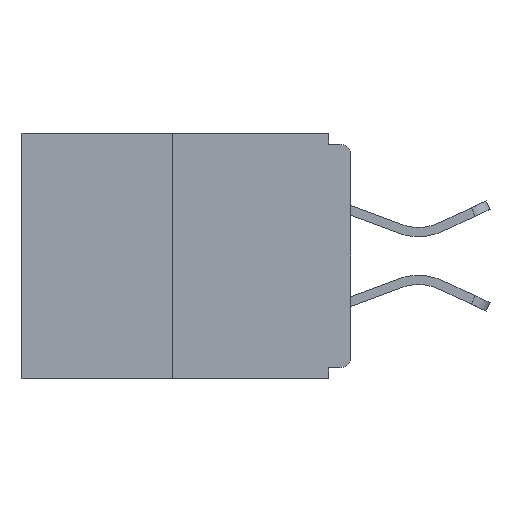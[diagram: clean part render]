
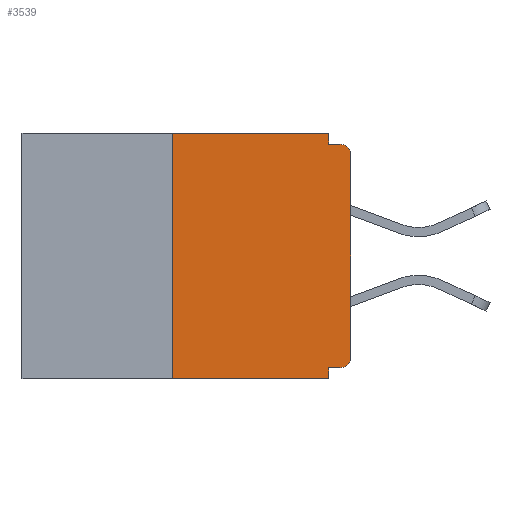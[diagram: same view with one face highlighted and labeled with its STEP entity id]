
A CAD part, left-side view. The second image highlights one B-rep face of the part: STEP entity #3539.
In plain terms, the highlighted planar face has unit normal (-1, 0, 0).
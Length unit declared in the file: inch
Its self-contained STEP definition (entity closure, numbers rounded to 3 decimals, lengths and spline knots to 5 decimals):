
#502 = CARTESIAN_POINT ( 'NONE',  ( 0., 0.46, 0. ) ) ;
#563 = EDGE_CURVE ( 'NONE', #7526, #619, #7329, .T. ) ;
#617 = CARTESIAN_POINT ( 'NONE',  ( 0., 0., 0. ) ) ;
#619 = VERTEX_POINT ( 'NONE', #12377 ) ;
#765 = DIRECTION ( 'NONE',  ( 0., 0., 1. ) ) ;
#1009 = CARTESIAN_POINT ( 'NONE',  ( 0., 0.031, -0.343 ) ) ;
#1024 = EDGE_CURVE ( 'NONE', #7980, #8264, #1423, .T. ) ;
#1290 = ORIENTED_EDGE ( 'NONE', *, *, #9973, .T. ) ;
#1423 = CIRCLE ( 'NONE', #4013, 0.015 ) ;
#1429 = CARTESIAN_POINT ( 'NONE',  ( 0., 0.031, -0.343 ) ) ;
#1476 = ORIENTED_EDGE ( 'NONE', *, *, #5410, .F. ) ;
#1592 = VECTOR ( 'NONE', #1594, 39.37008 ) ;
#1594 = DIRECTION ( 'NONE',  ( 0., 1., 0. ) ) ;
#1941 = DIRECTION ( 'NONE',  ( -1., 0., 0. ) ) ;
#1997 = CARTESIAN_POINT ( 'NONE',  ( 0., 0.46, -0.343 ) ) ;
#2198 = CARTESIAN_POINT ( 'NONE',  ( 0., 0.031, 0. ) ) ;
#2380 = VECTOR ( 'NONE', #7196, 39.37008 ) ;
#2473 = CARTESIAN_POINT ( 'NONE',  ( 0., 0.015, -0.328 ) ) ;
#2651 = VERTEX_POINT ( 'NONE', #6211 ) ;
#2707 = VECTOR ( 'NONE', #7493, 39.37008 ) ;
#2722 = DIRECTION ( 'NONE',  ( 0., -1., 0. ) ) ;
#2783 = LINE ( 'NONE', #9301, #4203 ) ;
#2908 = CARTESIAN_POINT ( 'NONE',  ( 0., 0., -0.03 ) ) ;
#3265 = PLANE ( 'NONE',  #10015 ) ;
#3532 = CARTESIAN_POINT ( 'NONE',  ( 0., 0.015, -0.015 ) ) ;
#3539 = ADVANCED_FACE ( 'NONE', ( #5276 ), #3265, .F. ) ;
#3884 = ORIENTED_EDGE ( 'NONE', *, *, #563, .F. ) ;
#3945 = CARTESIAN_POINT ( 'NONE',  ( 0., 0.015, -0.03 ) ) ;
#3946 = CARTESIAN_POINT ( 'NONE',  ( 0., 0.031, 0. ) ) ;
#4000 = ORIENTED_EDGE ( 'NONE', *, *, #6491, .F. ) ;
#4013 = AXIS2_PLACEMENT_3D ( 'NONE', #5721, #1941, #5534 ) ;
#4203 = VECTOR ( 'NONE', #2722, 39.37008 ) ;
#4237 = CARTESIAN_POINT ( 'NONE',  ( 0., 0.031, -0.015 ) ) ;
#4434 = VERTEX_POINT ( 'NONE', #2198 ) ;
#4523 = EDGE_CURVE ( 'NONE', #619, #4434, #6248, .T. ) ;
#4930 = VECTOR ( 'NONE', #6283, 39.37008 ) ;
#5276 = FACE_OUTER_BOUND ( 'NONE', #11549, .T. ) ;
#5347 = CARTESIAN_POINT ( 'NONE',  ( 0., 0.46, 0. ) ) ;
#5410 = EDGE_CURVE ( 'NONE', #4434, #6881, #11547, .T. ) ;
#5431 = VERTEX_POINT ( 'NONE', #1009 ) ;
#5495 = CARTESIAN_POINT ( 'NONE',  ( 0., 0.25, -0.343 ) ) ;
#5534 = DIRECTION ( 'NONE',  ( 0., 0., -1. ) ) ;
#5581 = EDGE_CURVE ( 'NONE', #8264, #8091, #8442, .T. ) ;
#5721 = CARTESIAN_POINT ( 'NONE',  ( 0., 0.015, -0.313 ) ) ;
#5841 = LINE ( 'NONE', #1997, #8376 ) ;
#6211 = CARTESIAN_POINT ( 'NONE',  ( 0., 0.031, -0.328 ) ) ;
#6248 = LINE ( 'NONE', #502, #2380 ) ;
#6283 = DIRECTION ( 'NONE',  ( 0., 0., -1. ) ) ;
#6317 = EDGE_CURVE ( 'NONE', #7526, #5431, #5841, .T. ) ;
#6377 = CARTESIAN_POINT ( 'NONE',  ( 0., 0.25, 0. ) ) ;
#6491 = EDGE_CURVE ( 'NONE', #2651, #5431, #7106, .T. ) ;
#6863 = ORIENTED_EDGE ( 'NONE', *, *, #1024, .T. ) ;
#6881 = VERTEX_POINT ( 'NONE', #4237 ) ;
#6910 = VERTEX_POINT ( 'NONE', #3532 ) ;
#7106 = LINE ( 'NONE', #1429, #4930 ) ;
#7196 = DIRECTION ( 'NONE',  ( 0., -1., 0. ) ) ;
#7329 = LINE ( 'NONE', #6377, #10081 ) ;
#7493 = DIRECTION ( 'NONE',  ( 0., 0., 1. ) ) ;
#7526 = VERTEX_POINT ( 'NONE', #5495 ) ;
#7821 = DIRECTION ( 'NONE',  ( 0., 0., -1. ) ) ;
#7980 = VERTEX_POINT ( 'NONE', #2473 ) ;
#8091 = VERTEX_POINT ( 'NONE', #2908 ) ;
#8264 = VERTEX_POINT ( 'NONE', #10999 ) ;
#8376 = VECTOR ( 'NONE', #10748, 39.37008 ) ;
#8391 = LINE ( 'NONE', #9409, #1592 ) ;
#8442 = LINE ( 'NONE', #617, #2707 ) ;
#8586 = CIRCLE ( 'NONE', #9596, 0.015 ) ;
#9151 = DIRECTION ( 'NONE',  ( 0., 0., -1. ) ) ;
#9166 = ORIENTED_EDGE ( 'NONE', *, *, #9200, .F. ) ;
#9200 = EDGE_CURVE ( 'NONE', #7980, #2651, #8391, .T. ) ;
#9216 = VECTOR ( 'NONE', #7821, 39.37008 ) ;
#9301 = CARTESIAN_POINT ( 'NONE',  ( 0., 0., -0.015 ) ) ;
#9409 = CARTESIAN_POINT ( 'NONE',  ( 0., 0., -0.328 ) ) ;
#9530 = ORIENTED_EDGE ( 'NONE', *, *, #5581, .T. ) ;
#9596 = AXIS2_PLACEMENT_3D ( 'NONE', #3945, #11546, #10710 ) ;
#9973 = EDGE_CURVE ( 'NONE', #8091, #6910, #8586, .T. ) ;
#10015 = AXIS2_PLACEMENT_3D ( 'NONE', #5347, #10968, #9151 ) ;
#10081 = VECTOR ( 'NONE', #765, 39.37008 ) ;
#10127 = ORIENTED_EDGE ( 'NONE', *, *, #10641, .F. ) ;
#10206 = ORIENTED_EDGE ( 'NONE', *, *, #4523, .F. ) ;
#10641 = EDGE_CURVE ( 'NONE', #6881, #6910, #2783, .T. ) ;
#10710 = DIRECTION ( 'NONE',  ( 0., 0., -1. ) ) ;
#10748 = DIRECTION ( 'NONE',  ( 0., -1., 0. ) ) ;
#10968 = DIRECTION ( 'NONE',  ( 1., 0., 0. ) ) ;
#10999 = CARTESIAN_POINT ( 'NONE',  ( 0., 0., -0.313 ) ) ;
#11546 = DIRECTION ( 'NONE',  ( -1., 0., 0. ) ) ;
#11547 = LINE ( 'NONE', #3946, #9216 ) ;
#11549 = EDGE_LOOP ( 'NONE', ( #10206, #3884, #12394, #4000, #9166, #6863, #9530, #1290, #10127, #1476 ) ) ;
#12377 = CARTESIAN_POINT ( 'NONE',  ( 0., 0.25, 0. ) ) ;
#12394 = ORIENTED_EDGE ( 'NONE', *, *, #6317, .T. ) ;
